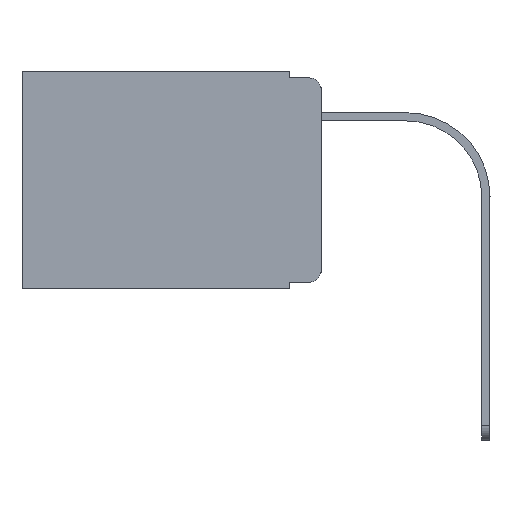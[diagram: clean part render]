
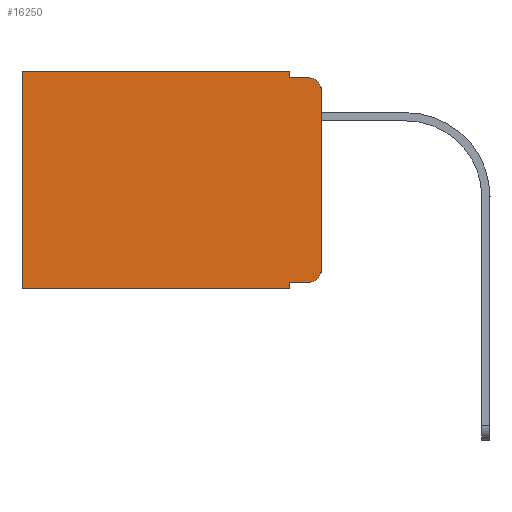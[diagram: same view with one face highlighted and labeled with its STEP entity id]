
A CAD part, left-side view. The second image highlights one B-rep face of the part: STEP entity #16250.
In plain terms, the highlighted planar face has unit normal (-1, 0, 0).
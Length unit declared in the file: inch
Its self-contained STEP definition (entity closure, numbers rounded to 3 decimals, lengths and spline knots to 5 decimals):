
#76 = VERTEX_POINT ( 'NONE', #15060 ) ;
#545 = EDGE_CURVE ( 'NONE', #1823, #8572, #15360, .T. ) ;
#719 = VECTOR ( 'NONE', #5345, 39.37008 ) ;
#791 = VERTEX_POINT ( 'NONE', #16009 ) ;
#957 = DIRECTION ( 'NONE',  ( 0., -1., 0. ) ) ;
#979 = CARTESIAN_POINT ( 'NONE',  ( 0.298, 0., -0.313 ) ) ;
#1057 = CARTESIAN_POINT ( 'NONE',  ( 0.298, 0.051, 0. ) ) ;
#1113 = EDGE_LOOP ( 'NONE', ( #1654, #5942, #15623, #5366, #4941, #16428, #1919, #7473, #5200, #8529 ) ) ;
#1256 = VECTOR ( 'NONE', #12570, 39.37008 ) ;
#1593 = CARTESIAN_POINT ( 'NONE',  ( 0.298, 0., -0.343 ) ) ;
#1654 = ORIENTED_EDGE ( 'NONE', *, *, #5966, .F. ) ;
#1823 = VERTEX_POINT ( 'NONE', #8600 ) ;
#1919 = ORIENTED_EDGE ( 'NONE', *, *, #8883, .F. ) ;
#1958 = VERTEX_POINT ( 'NONE', #11813 ) ;
#2045 = VECTOR ( 'NONE', #8828, 39.37008 ) ;
#2049 = CARTESIAN_POINT ( 'NONE',  ( 0.298, 0., 0. ) ) ;
#2931 = VERTEX_POINT ( 'NONE', #979 ) ;
#2932 = EDGE_CURVE ( 'NONE', #76, #14843, #11390, .T. ) ;
#2996 = CARTESIAN_POINT ( 'NONE',  ( 0.298, 0.02, -0.01 ) ) ;
#3143 = EDGE_CURVE ( 'NONE', #1823, #791, #16718, .T. ) ;
#3156 = PLANE ( 'NONE',  #5567 ) ;
#3211 = DIRECTION ( 'NONE',  ( 0., 1., 0. ) ) ;
#3379 = EDGE_CURVE ( 'NONE', #14843, #14513, #4597, .T. ) ;
#3759 = DIRECTION ( 'NONE',  ( 0., -1., 0. ) ) ;
#4091 = LINE ( 'NONE', #10523, #719 ) ;
#4597 = LINE ( 'NONE', #14924, #5053 ) ;
#4599 = VECTOR ( 'NONE', #3759, 39.37008 ) ;
#4657 = DIRECTION ( 'NONE',  ( 0., 0., -1. ) ) ;
#4941 = ORIENTED_EDGE ( 'NONE', *, *, #6904, .T. ) ;
#5053 = VECTOR ( 'NONE', #957, 39.37008 ) ;
#5200 = ORIENTED_EDGE ( 'NONE', *, *, #545, .T. ) ;
#5345 = DIRECTION ( 'NONE',  ( 0., 0., -1. ) ) ;
#5366 = ORIENTED_EDGE ( 'NONE', *, *, #2932, .F. ) ;
#5567 = AXIS2_PLACEMENT_3D ( 'NONE', #8310, #7042, #4657 ) ;
#5942 = ORIENTED_EDGE ( 'NONE', *, *, #9585, .T. ) ;
#5966 = EDGE_CURVE ( 'NONE', #7136, #2931, #4091, .T. ) ;
#6016 = AXIS2_PLACEMENT_3D ( 'NONE', #9159, #14386, #11943 ) ;
#6371 = CARTESIAN_POINT ( 'NONE',  ( 0.298, 0.051, -0.333 ) ) ;
#6904 = EDGE_CURVE ( 'NONE', #76, #11265, #12363, .T. ) ;
#7042 = DIRECTION ( 'NONE',  ( 1., 0., 0. ) ) ;
#7136 = VERTEX_POINT ( 'NONE', #13200 ) ;
#7473 = ORIENTED_EDGE ( 'NONE', *, *, #3143, .F. ) ;
#7933 = AXIS2_PLACEMENT_3D ( 'NONE', #14819, #8214, #13377 ) ;
#8175 = CARTESIAN_POINT ( 'NONE',  ( 0.298, 0.473, 0. ) ) ;
#8214 = DIRECTION ( 'NONE',  ( -1., 0., 0. ) ) ;
#8310 = CARTESIAN_POINT ( 'NONE',  ( 0.298, 0., 0. ) ) ;
#8529 = ORIENTED_EDGE ( 'NONE', *, *, #9791, .T. ) ;
#8572 = VERTEX_POINT ( 'NONE', #16244 ) ;
#8600 = CARTESIAN_POINT ( 'NONE',  ( 0.298, 0.051, -0.333 ) ) ;
#8828 = DIRECTION ( 'NONE',  ( 0., 1., 0. ) ) ;
#8883 = EDGE_CURVE ( 'NONE', #791, #1958, #9306, .T. ) ;
#9159 = CARTESIAN_POINT ( 'NONE',  ( 0.298, 0.02, -0.03 ) ) ;
#9306 = LINE ( 'NONE', #1593, #11677 ) ;
#9584 = FACE_OUTER_BOUND ( 'NONE', #1113, .T. ) ;
#9585 = EDGE_CURVE ( 'NONE', #7136, #14513, #15488, .T. ) ;
#9791 = EDGE_CURVE ( 'NONE', #8572, #2931, #13857, .T. ) ;
#10283 = DIRECTION ( 'NONE',  ( 0., 0., -1. ) ) ;
#10523 = CARTESIAN_POINT ( 'NONE',  ( 0.298, 0., 0. ) ) ;
#10730 = DIRECTION ( 'NONE',  ( 0., 0., -1. ) ) ;
#11133 = CARTESIAN_POINT ( 'NONE',  ( 0.298, 0.473, 0. ) ) ;
#11207 = VECTOR ( 'NONE', #10730, 39.37008 ) ;
#11265 = VERTEX_POINT ( 'NONE', #11133 ) ;
#11390 = LINE ( 'NONE', #1057, #1256 ) ;
#11677 = VECTOR ( 'NONE', #3211, 39.37008 ) ;
#11813 = CARTESIAN_POINT ( 'NONE',  ( 0.298, 0.473, -0.343 ) ) ;
#11943 = DIRECTION ( 'NONE',  ( 0., 0., -1. ) ) ;
#12074 = LINE ( 'NONE', #8175, #11207 ) ;
#12363 = LINE ( 'NONE', #2049, #2045 ) ;
#12570 = DIRECTION ( 'NONE',  ( 0., 0., -1. ) ) ;
#12993 = EDGE_CURVE ( 'NONE', #11265, #1958, #12074, .T. ) ;
#13200 = CARTESIAN_POINT ( 'NONE',  ( 0.298, 0., -0.03 ) ) ;
#13377 = DIRECTION ( 'NONE',  ( 0., 0., -1. ) ) ;
#13857 = CIRCLE ( 'NONE', #7933, 0.02 ) ;
#14256 = CARTESIAN_POINT ( 'NONE',  ( 0.298, 0.051, 0. ) ) ;
#14370 = CARTESIAN_POINT ( 'NONE',  ( 0.298, 0.051, -0.01 ) ) ;
#14386 = DIRECTION ( 'NONE',  ( -1., 0., 0. ) ) ;
#14513 = VERTEX_POINT ( 'NONE', #2996 ) ;
#14819 = CARTESIAN_POINT ( 'NONE',  ( 0.298, 0.02, -0.313 ) ) ;
#14843 = VERTEX_POINT ( 'NONE', #14370 ) ;
#14924 = CARTESIAN_POINT ( 'NONE',  ( 0.298, 0.051, -0.01 ) ) ;
#15060 = CARTESIAN_POINT ( 'NONE',  ( 0.298, 0.051, 0. ) ) ;
#15360 = LINE ( 'NONE', #6371, #4599 ) ;
#15488 = CIRCLE ( 'NONE', #6016, 0.02 ) ;
#15623 = ORIENTED_EDGE ( 'NONE', *, *, #3379, .F. ) ;
#15872 = VECTOR ( 'NONE', #10283, 39.37008 ) ;
#16009 = CARTESIAN_POINT ( 'NONE',  ( 0.298, 0.051, -0.343 ) ) ;
#16244 = CARTESIAN_POINT ( 'NONE',  ( 0.298, 0.02, -0.333 ) ) ;
#16250 = ADVANCED_FACE ( 'NONE', ( #9584 ), #3156, .F. ) ;
#16428 = ORIENTED_EDGE ( 'NONE', *, *, #12993, .T. ) ;
#16718 = LINE ( 'NONE', #14256, #15872 ) ;
